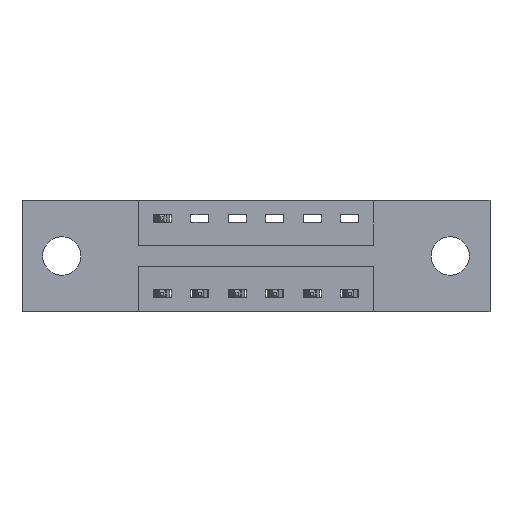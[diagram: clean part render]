
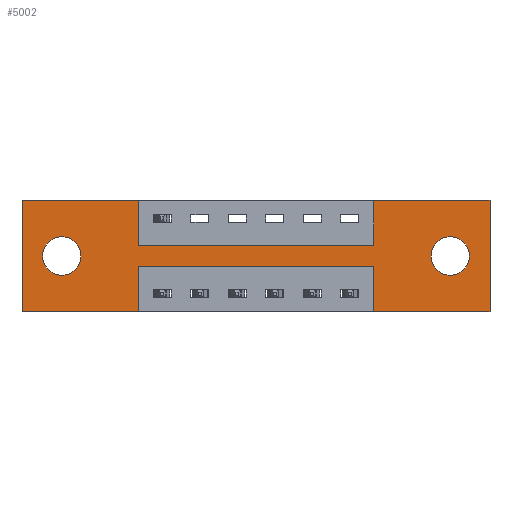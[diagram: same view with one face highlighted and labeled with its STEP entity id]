
A CAD part, front view. The second image highlights one B-rep face of the part: STEP entity #5002.
In plain terms, the highlighted planar face has unit normal (0, -1, 0).
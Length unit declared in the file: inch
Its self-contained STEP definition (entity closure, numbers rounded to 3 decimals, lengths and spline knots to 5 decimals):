
#14 = CARTESIAN_POINT ( 'NONE',  ( 1.56, 0., -0.37 ) ) ;
#57 = EDGE_LOOP ( 'NONE', ( #1118, #432, #6900, #7077, #7422, #4622, #1904, #655, #7921, #8255, #313, #7937 ) ) ;
#78 = LINE ( 'NONE', #6107, #1891 ) ;
#89 = CARTESIAN_POINT ( 'NONE',  ( 0., 0., 0. ) ) ;
#189 = CARTESIAN_POINT ( 'NONE',  ( 0.3875, 0., -0.22 ) ) ;
#250 = VERTEX_POINT ( 'NONE', #6200 ) ;
#311 = ORIENTED_EDGE ( 'NONE', *, *, #7903, .T. ) ;
#313 = ORIENTED_EDGE ( 'NONE', *, *, #3358, .F. ) ;
#332 = EDGE_CURVE ( 'NONE', #3965, #2895, #4783, .T. ) ;
#350 = CARTESIAN_POINT ( 'NONE',  ( 0.1325, 0., -0.249 ) ) ;
#398 = DIRECTION ( 'NONE',  ( 0., 0., -1. ) ) ;
#432 = ORIENTED_EDGE ( 'NONE', *, *, #7168, .F. ) ;
#452 = CARTESIAN_POINT ( 'NONE',  ( 1.1725, 0., 0. ) ) ;
#461 = VERTEX_POINT ( 'NONE', #89 ) ;
#477 = CIRCLE ( 'NONE', #1448, 0.064 ) ;
#510 = CARTESIAN_POINT ( 'NONE',  ( 1.1725, 0., -0.22 ) ) ;
#614 = DIRECTION ( 'NONE',  ( 0., 0., -1. ) ) ;
#644 = DIRECTION ( 'NONE',  ( 1., 0., 0. ) ) ;
#655 = ORIENTED_EDGE ( 'NONE', *, *, #5115, .F. ) ;
#674 = EDGE_CURVE ( 'NONE', #461, #3467, #2470, .T. ) ;
#773 = CARTESIAN_POINT ( 'NONE',  ( 0., 0., -0.37 ) ) ;
#853 = VECTOR ( 'NONE', #4395, 39.37008 ) ;
#959 = ORIENTED_EDGE ( 'NONE', *, *, #8183, .T. ) ;
#969 = LINE ( 'NONE', #3409, #6133 ) ;
#992 = CARTESIAN_POINT ( 'NONE',  ( 0.3875, 0., 0. ) ) ;
#1078 = CARTESIAN_POINT ( 'NONE',  ( 1.56, 0., 0. ) ) ;
#1118 = ORIENTED_EDGE ( 'NONE', *, *, #4735, .F. ) ;
#1156 = FACE_OUTER_BOUND ( 'NONE', #57, .T. ) ;
#1204 = VERTEX_POINT ( 'NONE', #7092 ) ;
#1252 = LINE ( 'NONE', #2143, #4634 ) ;
#1274 = EDGE_CURVE ( 'NONE', #3467, #1204, #2987, .T. ) ;
#1306 = CARTESIAN_POINT ( 'NONE',  ( 1.1725, 0., -0.15 ) ) ;
#1368 = VECTOR ( 'NONE', #4182, 39.37008 ) ;
#1394 = EDGE_CURVE ( 'NONE', #2895, #5123, #78, .T. ) ;
#1427 = DIRECTION ( 'NONE',  ( 0., 0., -1. ) ) ;
#1448 = AXIS2_PLACEMENT_3D ( 'NONE', #6131, #2104, #6771 ) ;
#1539 = CIRCLE ( 'NONE', #4902, 0.064 ) ;
#1645 = DIRECTION ( 'NONE',  ( 0., 1., 0. ) ) ;
#1765 = DIRECTION ( 'NONE',  ( 0., 1., 0. ) ) ;
#1766 = LINE ( 'NONE', #7633, #2966 ) ;
#1816 = CARTESIAN_POINT ( 'NONE',  ( 1.4275, 0., -0.249 ) ) ;
#1854 = CARTESIAN_POINT ( 'NONE',  ( 1.4275, 0., -0.185 ) ) ;
#1884 = VERTEX_POINT ( 'NONE', #2736 ) ;
#1891 = VECTOR ( 'NONE', #7012, 39.37008 ) ;
#1904 = ORIENTED_EDGE ( 'NONE', *, *, #8329, .F. ) ;
#1953 = EDGE_LOOP ( 'NONE', ( #959, #6637 ) ) ;
#2044 = VERTEX_POINT ( 'NONE', #1816 ) ;
#2104 = DIRECTION ( 'NONE',  ( 0., 1., 0. ) ) ;
#2143 = CARTESIAN_POINT ( 'NONE',  ( 0.3875, 0., -0.22 ) ) ;
#2288 = VERTEX_POINT ( 'NONE', #1078 ) ;
#2294 = ORIENTED_EDGE ( 'NONE', *, *, #7347, .T. ) ;
#2470 = LINE ( 'NONE', #5326, #853 ) ;
#2530 = AXIS2_PLACEMENT_3D ( 'NONE', #3114, #7713, #3797 ) ;
#2658 = CARTESIAN_POINT ( 'NONE',  ( 1.56, 0., 0. ) ) ;
#2736 = CARTESIAN_POINT ( 'NONE',  ( 0.3875, 0., -0.37 ) ) ;
#2778 = VECTOR ( 'NONE', #1427, 39.37008 ) ;
#2850 = DIRECTION ( 'NONE',  ( 0., 1., 0. ) ) ;
#2895 = VERTEX_POINT ( 'NONE', #6518 ) ;
#2919 = VERTEX_POINT ( 'NONE', #8288 ) ;
#2966 = VECTOR ( 'NONE', #7815, 39.37008 ) ;
#2984 = FACE_BOUND ( 'NONE', #8354, .T. ) ;
#2987 = LINE ( 'NONE', #3586, #2778 ) ;
#3114 = CARTESIAN_POINT ( 'NONE',  ( 0., 0., -0.37 ) ) ;
#3161 = AXIS2_PLACEMENT_3D ( 'NONE', #5685, #1645, #6348 ) ;
#3229 = CARTESIAN_POINT ( 'NONE',  ( 0.3875, 0., -0.15 ) ) ;
#3310 = DIRECTION ( 'NONE',  ( 0., 0., 1. ) ) ;
#3358 = EDGE_CURVE ( 'NONE', #2919, #461, #1766, .T. ) ;
#3409 = CARTESIAN_POINT ( 'NONE',  ( 0., 0., 0. ) ) ;
#3464 = CARTESIAN_POINT ( 'NONE',  ( 0.3875, 0., -0.37 ) ) ;
#3467 = VERTEX_POINT ( 'NONE', #992 ) ;
#3502 = EDGE_CURVE ( 'NONE', #2044, #6231, #6089, .T. ) ;
#3586 = CARTESIAN_POINT ( 'NONE',  ( 0.3875, 0., 0. ) ) ;
#3596 = DIRECTION ( 'NONE',  ( -1., 0., 0. ) ) ;
#3675 = EDGE_CURVE ( 'NONE', #6842, #2288, #969, .T. ) ;
#3797 = DIRECTION ( 'NONE',  ( 0., 0., -1. ) ) ;
#3891 = LINE ( 'NONE', #7237, #5435 ) ;
#3897 = VERTEX_POINT ( 'NONE', #1306 ) ;
#3935 = LINE ( 'NONE', #3229, #5479 ) ;
#3965 = VERTEX_POINT ( 'NONE', #14 ) ;
#4182 = DIRECTION ( 'NONE',  ( -1., 0., 0. ) ) ;
#4395 = DIRECTION ( 'NONE',  ( 1., 0., 0. ) ) ;
#4488 = VERTEX_POINT ( 'NONE', #350 ) ;
#4622 = ORIENTED_EDGE ( 'NONE', *, *, #3675, .F. ) ;
#4634 = VECTOR ( 'NONE', #4827, 39.37008 ) ;
#4735 = EDGE_CURVE ( 'NONE', #8035, #1884, #7211, .T. ) ;
#4768 = FACE_BOUND ( 'NONE', #1953, .T. ) ;
#4783 = LINE ( 'NONE', #5440, #8036 ) ;
#4827 = DIRECTION ( 'NONE',  ( -1., 0., 0. ) ) ;
#4902 = AXIS2_PLACEMENT_3D ( 'NONE', #5802, #1765, #6460 ) ;
#5002 = ADVANCED_FACE ( 'NONE', ( #4768, #2984, #1156 ), #5753, .T. ) ;
#5115 = EDGE_CURVE ( 'NONE', #1204, #3897, #3935, .T. ) ;
#5123 = VERTEX_POINT ( 'NONE', #510 ) ;
#5277 = VECTOR ( 'NONE', #7402, 39.37008 ) ;
#5326 = CARTESIAN_POINT ( 'NONE',  ( 0., 0., 0. ) ) ;
#5435 = VECTOR ( 'NONE', #3310, 39.37008 ) ;
#5440 = CARTESIAN_POINT ( 'NONE',  ( 0., 0., -0.37 ) ) ;
#5479 = VECTOR ( 'NONE', #8474, 39.37008 ) ;
#5685 = CARTESIAN_POINT ( 'NONE',  ( 0.1325, 0., -0.185 ) ) ;
#5753 = PLANE ( 'NONE',  #2530 ) ;
#5756 = AXIS2_PLACEMENT_3D ( 'NONE', #1854, #2850, #398 ) ;
#5802 = CARTESIAN_POINT ( 'NONE',  ( 1.4275, 0., -0.185 ) ) ;
#6089 = CIRCLE ( 'NONE', #5756, 0.064 ) ;
#6107 = CARTESIAN_POINT ( 'NONE',  ( 1.1725, 0., -0.37 ) ) ;
#6131 = CARTESIAN_POINT ( 'NONE',  ( 0.1325, 0., -0.185 ) ) ;
#6133 = VECTOR ( 'NONE', #644, 39.37008 ) ;
#6200 = CARTESIAN_POINT ( 'NONE',  ( 0.1325, 0., -0.121 ) ) ;
#6231 = VERTEX_POINT ( 'NONE', #7117 ) ;
#6348 = DIRECTION ( 'NONE',  ( 0., 0., 1. ) ) ;
#6460 = DIRECTION ( 'NONE',  ( 0., 0., -1. ) ) ;
#6518 = CARTESIAN_POINT ( 'NONE',  ( 1.1725, 0., -0.37 ) ) ;
#6535 = EDGE_CURVE ( 'NONE', #1884, #2919, #6888, .T. ) ;
#6637 = ORIENTED_EDGE ( 'NONE', *, *, #3502, .T. ) ;
#6759 = VECTOR ( 'NONE', #614, 39.37008 ) ;
#6771 = DIRECTION ( 'NONE',  ( 0., 0., 1. ) ) ;
#6842 = VERTEX_POINT ( 'NONE', #452 ) ;
#6888 = LINE ( 'NONE', #773, #1368 ) ;
#6900 = ORIENTED_EDGE ( 'NONE', *, *, #1394, .F. ) ;
#7012 = DIRECTION ( 'NONE',  ( 0., 0., 1. ) ) ;
#7077 = ORIENTED_EDGE ( 'NONE', *, *, #332, .F. ) ;
#7092 = CARTESIAN_POINT ( 'NONE',  ( 0.3875, 0., -0.15 ) ) ;
#7117 = CARTESIAN_POINT ( 'NONE',  ( 1.4275, 0., -0.121 ) ) ;
#7168 = EDGE_CURVE ( 'NONE', #5123, #8035, #1252, .T. ) ;
#7211 = LINE ( 'NONE', #3464, #5277 ) ;
#7237 = CARTESIAN_POINT ( 'NONE',  ( 1.1725, 0., 0. ) ) ;
#7347 = EDGE_CURVE ( 'NONE', #4488, #250, #8397, .T. ) ;
#7402 = DIRECTION ( 'NONE',  ( 0., 0., -1. ) ) ;
#7422 = ORIENTED_EDGE ( 'NONE', *, *, #8368, .F. ) ;
#7633 = CARTESIAN_POINT ( 'NONE',  ( 0., 0., 0. ) ) ;
#7713 = DIRECTION ( 'NONE',  ( 0., -1., 0. ) ) ;
#7815 = DIRECTION ( 'NONE',  ( 0., 0., 1. ) ) ;
#7903 = EDGE_CURVE ( 'NONE', #250, #4488, #477, .T. ) ;
#7921 = ORIENTED_EDGE ( 'NONE', *, *, #1274, .F. ) ;
#7937 = ORIENTED_EDGE ( 'NONE', *, *, #6535, .F. ) ;
#8035 = VERTEX_POINT ( 'NONE', #189 ) ;
#8036 = VECTOR ( 'NONE', #3596, 39.37008 ) ;
#8183 = EDGE_CURVE ( 'NONE', #6231, #2044, #1539, .T. ) ;
#8255 = ORIENTED_EDGE ( 'NONE', *, *, #674, .F. ) ;
#8288 = CARTESIAN_POINT ( 'NONE',  ( 0., 0., -0.37 ) ) ;
#8329 = EDGE_CURVE ( 'NONE', #3897, #6842, #3891, .T. ) ;
#8354 = EDGE_LOOP ( 'NONE', ( #311, #2294 ) ) ;
#8368 = EDGE_CURVE ( 'NONE', #2288, #3965, #8479, .T. ) ;
#8397 = CIRCLE ( 'NONE', #3161, 0.064 ) ;
#8474 = DIRECTION ( 'NONE',  ( 1., 0., 0. ) ) ;
#8479 = LINE ( 'NONE', #2658, #6759 ) ;
